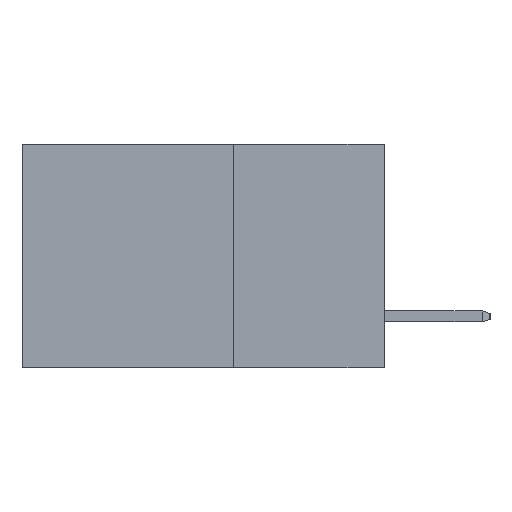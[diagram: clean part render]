
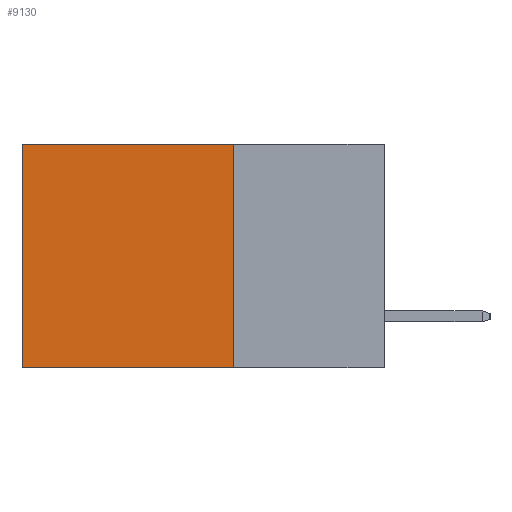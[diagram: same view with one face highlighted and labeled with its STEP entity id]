
A CAD part, left-side view. The second image highlights one B-rep face of the part: STEP entity #9130.
In plain terms, the highlighted planar face has unit normal (-1, 0, 0).
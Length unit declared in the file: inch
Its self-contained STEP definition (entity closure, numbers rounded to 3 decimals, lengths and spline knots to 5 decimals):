
#45 = CARTESIAN_POINT ( 'NONE',  ( 0.2615, 0.6, -0.37 ) ) ;
#71 = CARTESIAN_POINT ( 'NONE',  ( 0.2615, 0.25, -0.37 ) ) ;
#357 = ORIENTED_EDGE ( 'NONE', *, *, #7932, .T. ) ;
#1614 = VECTOR ( 'NONE', #8963, 39.37008 ) ;
#2374 = LINE ( 'NONE', #5474, #4105 ) ;
#2377 = DIRECTION ( 'NONE',  ( 0., 0., -1. ) ) ;
#2447 = CARTESIAN_POINT ( 'NONE',  ( 0.2615, 0.25, -0.37 ) ) ;
#3840 = CARTESIAN_POINT ( 'NONE',  ( 0.2615, 0.6, -0.37 ) ) ;
#4105 = VECTOR ( 'NONE', #4758, 39.37008 ) ;
#4288 = FACE_OUTER_BOUND ( 'NONE', #6493, .T. ) ;
#4431 = ORIENTED_EDGE ( 'NONE', *, *, #5674, .F. ) ;
#4520 = DIRECTION ( 'NONE',  ( 0., 0., -1. ) ) ;
#4758 = DIRECTION ( 'NONE',  ( 0., 1., 0. ) ) ;
#5451 = DIRECTION ( 'NONE',  ( 0., 1., 0. ) ) ;
#5474 = CARTESIAN_POINT ( 'NONE',  ( 0.2615, 0.25, 0. ) ) ;
#5674 = EDGE_CURVE ( 'NONE', #6753, #7914, #5993, .T. ) ;
#5993 = LINE ( 'NONE', #2447, #9407 ) ;
#6256 = EDGE_CURVE ( 'NONE', #8391, #8121, #2374, .T. ) ;
#6338 = ORIENTED_EDGE ( 'NONE', *, *, #6256, .T. ) ;
#6493 = EDGE_LOOP ( 'NONE', ( #357, #4431, #8181, #6338 ) ) ;
#6753 = VERTEX_POINT ( 'NONE', #71 ) ;
#7211 = VECTOR ( 'NONE', #2377, 39.37008 ) ;
#7215 = AXIS2_PLACEMENT_3D ( 'NONE', #8198, #8928, #4520 ) ;
#7460 = PLANE ( 'NONE',  #7215 ) ;
#7530 = LINE ( 'NONE', #8993, #1614 ) ;
#7914 = VERTEX_POINT ( 'NONE', #45 ) ;
#7932 = EDGE_CURVE ( 'NONE', #8121, #7914, #9134, .T. ) ;
#8121 = VERTEX_POINT ( 'NONE', #8485 ) ;
#8181 = ORIENTED_EDGE ( 'NONE', *, *, #9189, .F. ) ;
#8198 = CARTESIAN_POINT ( 'NONE',  ( 0.2615, 0.25, -0.37 ) ) ;
#8391 = VERTEX_POINT ( 'NONE', #8784 ) ;
#8485 = CARTESIAN_POINT ( 'NONE',  ( 0.2615, 0.6, 0. ) ) ;
#8784 = CARTESIAN_POINT ( 'NONE',  ( 0.2615, 0.25, 0. ) ) ;
#8928 = DIRECTION ( 'NONE',  ( 1., 0., 0. ) ) ;
#8963 = DIRECTION ( 'NONE',  ( 0., 0., -1. ) ) ;
#8993 = CARTESIAN_POINT ( 'NONE',  ( 0.2615, 0.25, -0.37 ) ) ;
#9130 = ADVANCED_FACE ( 'NONE', ( #4288 ), #7460, .F. ) ;
#9134 = LINE ( 'NONE', #3840, #7211 ) ;
#9189 = EDGE_CURVE ( 'NONE', #8391, #6753, #7530, .T. ) ;
#9407 = VECTOR ( 'NONE', #5451, 39.37008 ) ;
